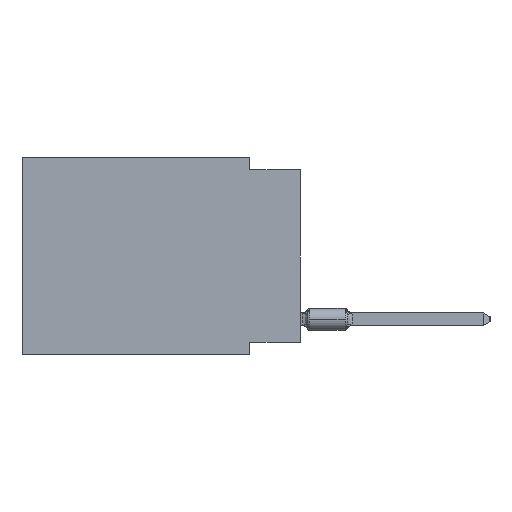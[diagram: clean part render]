
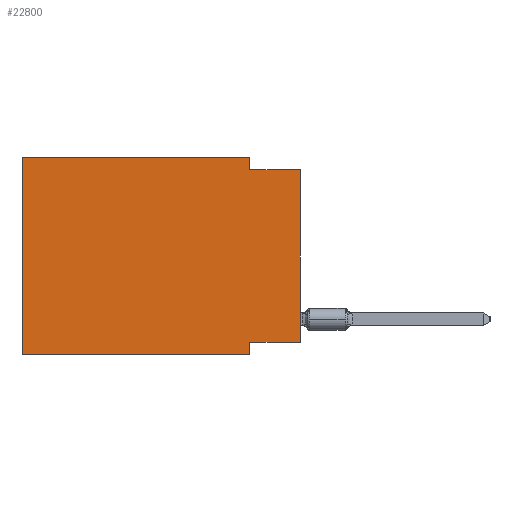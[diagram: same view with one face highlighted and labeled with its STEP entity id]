
A CAD part, left-side view. The second image highlights one B-rep face of the part: STEP entity #22800.
In plain terms, the highlighted planar face has unit normal (-1, 0, 0).
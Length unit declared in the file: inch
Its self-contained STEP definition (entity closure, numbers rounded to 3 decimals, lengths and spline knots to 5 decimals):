
#428 = CARTESIAN_POINT ( 'NONE',  ( 0., 0.1, 0. ) ) ;
#929 = DIRECTION ( 'NONE',  ( 0., 0., 1. ) ) ;
#1171 = VERTEX_POINT ( 'NONE', #2507 ) ;
#1300 = VECTOR ( 'NONE', #24377, 39.37008 ) ;
#2507 = CARTESIAN_POINT ( 'NONE',  ( 0., 0.55, -0.39 ) ) ;
#3734 = ORIENTED_EDGE ( 'NONE', *, *, #6185, .F. ) ;
#4165 = VECTOR ( 'NONE', #42421, 39.37008 ) ;
#4487 = AXIS2_PLACEMENT_3D ( 'NONE', #41218, #28227, #37857 ) ;
#6185 = EDGE_CURVE ( 'NONE', #1171, #41742, #29150, .T. ) ;
#8691 = VERTEX_POINT ( 'NONE', #41997 ) ;
#8782 = VERTEX_POINT ( 'NONE', #18694 ) ;
#9427 = DIRECTION ( 'NONE',  ( 0., -1., 0. ) ) ;
#9642 = EDGE_CURVE ( 'NONE', #1171, #8782, #29356, .T. ) ;
#10099 = ORIENTED_EDGE ( 'NONE', *, *, #20920, .F. ) ;
#11130 = VECTOR ( 'NONE', #12308, 39.37008 ) ;
#12308 = DIRECTION ( 'NONE',  ( 0., -1., 0. ) ) ;
#12495 = EDGE_CURVE ( 'NONE', #21232, #35681, #26473, .T. ) ;
#12779 = VECTOR ( 'NONE', #9427, 39.37008 ) ;
#13965 = CARTESIAN_POINT ( 'NONE',  ( 0., 0., -0.025 ) ) ;
#14321 = FACE_OUTER_BOUND ( 'NONE', #28398, .T. ) ;
#14640 = LINE ( 'NONE', #28099, #38044 ) ;
#14742 = ORIENTED_EDGE ( 'NONE', *, *, #15622, .F. ) ;
#15012 = CARTESIAN_POINT ( 'NONE',  ( 0., 0.1, 0. ) ) ;
#15622 = EDGE_CURVE ( 'NONE', #8691, #39491, #16338, .T. ) ;
#15685 = CARTESIAN_POINT ( 'NONE',  ( 0., 0.55, -0.39 ) ) ;
#16338 = LINE ( 'NONE', #36724, #38591 ) ;
#18132 = PLANE ( 'NONE',  #4487 ) ;
#18517 = EDGE_CURVE ( 'NONE', #39491, #8782, #25854, .T. ) ;
#18694 = CARTESIAN_POINT ( 'NONE',  ( 0., 0.1, -0.39 ) ) ;
#19616 = ORIENTED_EDGE ( 'NONE', *, *, #9642, .T. ) ;
#20920 = EDGE_CURVE ( 'NONE', #41742, #40920, #39741, .T. ) ;
#21232 = VERTEX_POINT ( 'NONE', #38116 ) ;
#21641 = CARTESIAN_POINT ( 'NONE',  ( 0., 0.55, 0. ) ) ;
#22800 = ADVANCED_FACE ( 'NONE', ( #14321 ), #18132, .F. ) ;
#22987 = VECTOR ( 'NONE', #929, 39.37008 ) ;
#24377 = DIRECTION ( 'NONE',  ( 0., 0., -1. ) ) ;
#25670 = LINE ( 'NONE', #428, #1300 ) ;
#25803 = ORIENTED_EDGE ( 'NONE', *, *, #28134, .T. ) ;
#25854 = LINE ( 'NONE', #39524, #38747 ) ;
#26473 = LINE ( 'NONE', #33612, #12779 ) ;
#26809 = ORIENTED_EDGE ( 'NONE', *, *, #37558, .F. ) ;
#28099 = CARTESIAN_POINT ( 'NONE',  ( 0., 0., 0. ) ) ;
#28134 = EDGE_CURVE ( 'NONE', #8691, #35681, #14640, .T. ) ;
#28227 = DIRECTION ( 'NONE',  ( 1., 0., 0. ) ) ;
#28398 = EDGE_LOOP ( 'NONE', ( #25803, #32089, #26809, #10099, #3734, #19616, #34267, #14742 ) ) ;
#29150 = LINE ( 'NONE', #41919, #22987 ) ;
#29356 = LINE ( 'NONE', #15685, #11130 ) ;
#29574 = DIRECTION ( 'NONE',  ( 0., 1., 0. ) ) ;
#32089 = ORIENTED_EDGE ( 'NONE', *, *, #12495, .F. ) ;
#32802 = DIRECTION ( 'NONE',  ( 0., 0., -1. ) ) ;
#33612 = CARTESIAN_POINT ( 'NONE',  ( 0., 0., -0.025 ) ) ;
#34267 = ORIENTED_EDGE ( 'NONE', *, *, #18517, .F. ) ;
#35681 = VERTEX_POINT ( 'NONE', #13965 ) ;
#36724 = CARTESIAN_POINT ( 'NONE',  ( 0., 0., -0.365 ) ) ;
#37558 = EDGE_CURVE ( 'NONE', #40920, #21232, #25670, .T. ) ;
#37857 = DIRECTION ( 'NONE',  ( 0., 0., -1. ) ) ;
#38044 = VECTOR ( 'NONE', #42194, 39.37008 ) ;
#38116 = CARTESIAN_POINT ( 'NONE',  ( 0., 0.1, -0.025 ) ) ;
#38591 = VECTOR ( 'NONE', #29574, 39.37008 ) ;
#38747 = VECTOR ( 'NONE', #32802, 39.37008 ) ;
#39072 = CARTESIAN_POINT ( 'NONE',  ( 0., 0.55, 0. ) ) ;
#39491 = VERTEX_POINT ( 'NONE', #43297 ) ;
#39524 = CARTESIAN_POINT ( 'NONE',  ( 0., 0.1, -0.39 ) ) ;
#39741 = LINE ( 'NONE', #39072, #4165 ) ;
#40920 = VERTEX_POINT ( 'NONE', #15012 ) ;
#41218 = CARTESIAN_POINT ( 'NONE',  ( 0., 0.55, 0. ) ) ;
#41742 = VERTEX_POINT ( 'NONE', #21641 ) ;
#41919 = CARTESIAN_POINT ( 'NONE',  ( 0., 0.55, 0. ) ) ;
#41997 = CARTESIAN_POINT ( 'NONE',  ( 0., 0., -0.365 ) ) ;
#42194 = DIRECTION ( 'NONE',  ( 0., 0., 1. ) ) ;
#42421 = DIRECTION ( 'NONE',  ( 0., -1., 0. ) ) ;
#43297 = CARTESIAN_POINT ( 'NONE',  ( 0., 0.1, -0.365 ) ) ;
